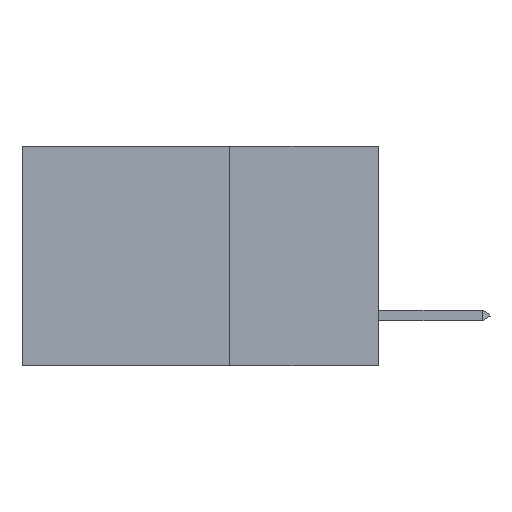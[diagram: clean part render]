
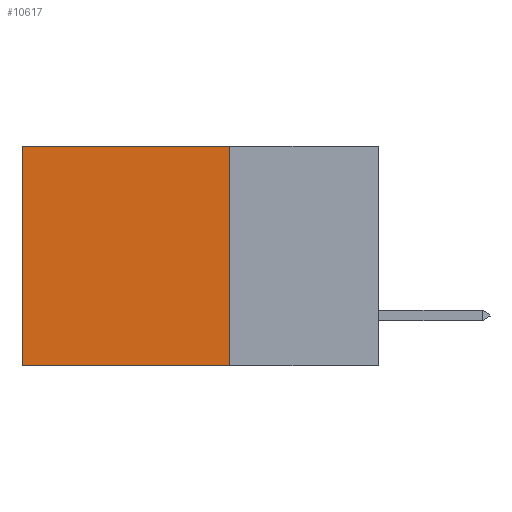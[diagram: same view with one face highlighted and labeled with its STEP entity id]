
A CAD part, left-side view. The second image highlights one B-rep face of the part: STEP entity #10617.
In plain terms, the highlighted planar face has unit normal (-1, 0, 0).
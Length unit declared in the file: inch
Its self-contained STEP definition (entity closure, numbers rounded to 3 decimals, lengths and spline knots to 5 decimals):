
#126 = CARTESIAN_POINT ( 'NONE',  ( 0.298, 0.25, 0. ) ) ;
#703 = EDGE_CURVE ( 'NONE', #8551, #15780, #8845, .T. ) ;
#1575 = CARTESIAN_POINT ( 'NONE',  ( 0.298, 0.6, 0. ) ) ;
#1869 = VERTEX_POINT ( 'NONE', #13986 ) ;
#2116 = DIRECTION ( 'NONE',  ( 0., 1., 0. ) ) ;
#2926 = DIRECTION ( 'NONE',  ( 0., 1., 0. ) ) ;
#3319 = DIRECTION ( 'NONE',  ( 0., 0., -1. ) ) ;
#4272 = EDGE_CURVE ( 'NONE', #19115, #1869, #6548, .T. ) ;
#6290 = ORIENTED_EDGE ( 'NONE', *, *, #21710, .T. ) ;
#6548 = LINE ( 'NONE', #13082, #17533 ) ;
#6727 = EDGE_CURVE ( 'NONE', #8551, #19115, #14775, .T. ) ;
#6898 = DIRECTION ( 'NONE',  ( 1., 0., 0. ) ) ;
#6973 = CARTESIAN_POINT ( 'NONE',  ( 0.298, 0.25, 0. ) ) ;
#7146 = VECTOR ( 'NONE', #3319, 39.37008 ) ;
#7333 = CARTESIAN_POINT ( 'NONE',  ( 0.298, 0.6, 0. ) ) ;
#8551 = VERTEX_POINT ( 'NONE', #6973 ) ;
#8752 = AXIS2_PLACEMENT_3D ( 'NONE', #20750, #6898, #20682 ) ;
#8845 = LINE ( 'NONE', #126, #17174 ) ;
#10617 = ADVANCED_FACE ( 'NONE', ( #16360 ), #18593, .F. ) ;
#11035 = DIRECTION ( 'NONE',  ( 0., 0., -1. ) ) ;
#11277 = VECTOR ( 'NONE', #11035, 39.37008 ) ;
#13082 = CARTESIAN_POINT ( 'NONE',  ( 0.298, 0.25, -0.37 ) ) ;
#13986 = CARTESIAN_POINT ( 'NONE',  ( 0.298, 0.6, -0.37 ) ) ;
#14201 = CARTESIAN_POINT ( 'NONE',  ( 0.298, 0.25, 0. ) ) ;
#14775 = LINE ( 'NONE', #14201, #11277 ) ;
#15780 = VERTEX_POINT ( 'NONE', #7333 ) ;
#16331 = ORIENTED_EDGE ( 'NONE', *, *, #4272, .F. ) ;
#16360 = FACE_OUTER_BOUND ( 'NONE', #20825, .T. ) ;
#16409 = ORIENTED_EDGE ( 'NONE', *, *, #6727, .F. ) ;
#16545 = ORIENTED_EDGE ( 'NONE', *, *, #703, .T. ) ;
#17174 = VECTOR ( 'NONE', #2116, 39.37008 ) ;
#17533 = VECTOR ( 'NONE', #2926, 39.37008 ) ;
#18593 = PLANE ( 'NONE',  #8752 ) ;
#19115 = VERTEX_POINT ( 'NONE', #21554 ) ;
#20682 = DIRECTION ( 'NONE',  ( 0., 0., -1. ) ) ;
#20750 = CARTESIAN_POINT ( 'NONE',  ( 0.298, 0.25, 0. ) ) ;
#20794 = LINE ( 'NONE', #1575, #7146 ) ;
#20825 = EDGE_LOOP ( 'NONE', ( #6290, #16331, #16409, #16545 ) ) ;
#21554 = CARTESIAN_POINT ( 'NONE',  ( 0.298, 0.25, -0.37 ) ) ;
#21710 = EDGE_CURVE ( 'NONE', #15780, #1869, #20794, .T. ) ;
